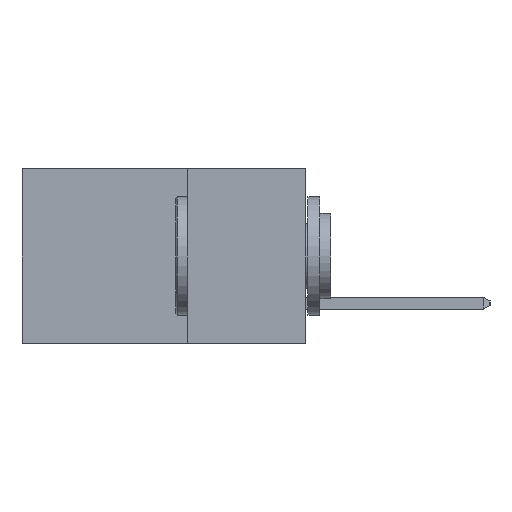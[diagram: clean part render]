
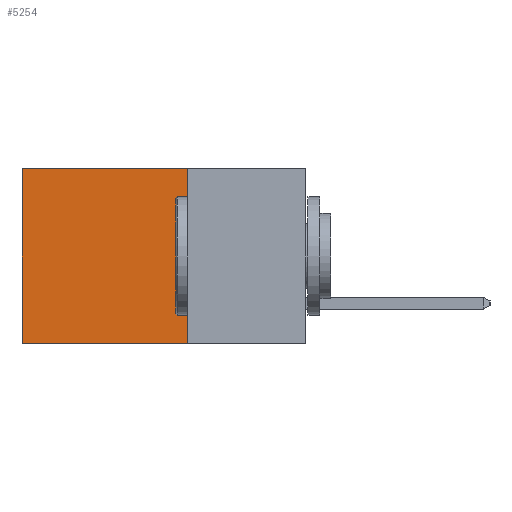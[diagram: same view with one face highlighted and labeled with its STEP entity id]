
A CAD part, left-side view. The second image highlights one B-rep face of the part: STEP entity #5254.
In plain terms, the highlighted planar face has unit normal (-1, 0, 0).
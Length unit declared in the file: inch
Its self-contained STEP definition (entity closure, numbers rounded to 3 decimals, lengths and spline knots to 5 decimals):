
#46 = CARTESIAN_POINT ( 'NONE',  ( 0.2615, 0.6, -0.37 ) ) ;
#59 = CARTESIAN_POINT ( 'NONE',  ( 0.2615, 0.25, 0. ) ) ;
#62 = DIRECTION ( 'NONE',  ( 0., 0., -1. ) ) ;
#90 = LINE ( 'NONE', #10344, #10865 ) ;
#105 = DIRECTION ( 'NONE',  ( 0., 1., 0. ) ) ;
#161 = DIRECTION ( 'NONE',  ( 1., 0., 0. ) ) ;
#405 = EDGE_LOOP ( 'NONE', ( #10939, #8614, #11248, #3374 ) ) ;
#822 = VECTOR ( 'NONE', #105, 39.37008 ) ;
#895 = VECTOR ( 'NONE', #6299, 39.37008 ) ;
#998 = PLANE ( 'NONE',  #1744 ) ;
#1107 = DIRECTION ( 'NONE',  ( 0., 0., -1. ) ) ;
#1227 = CARTESIAN_POINT ( 'NONE',  ( 0.2615, 0.25, -0.37 ) ) ;
#1744 = AXIS2_PLACEMENT_3D ( 'NONE', #1227, #161, #62 ) ;
#3213 = VERTEX_POINT ( 'NONE', #11982 ) ;
#3374 = ORIENTED_EDGE ( 'NONE', *, *, #8757, .T. ) ;
#4241 = CARTESIAN_POINT ( 'NONE',  ( 0.2615, 0.25, -0.37 ) ) ;
#5219 = VERTEX_POINT ( 'NONE', #4241 ) ;
#5245 = CARTESIAN_POINT ( 'NONE',  ( 0.2615, 0.25, -0.37 ) ) ;
#5254 = ADVANCED_FACE ( 'NONE', ( #10800 ), #998, .F. ) ;
#5263 = EDGE_CURVE ( 'NONE', #5577, #6019, #5347, .T. ) ;
#5347 = LINE ( 'NONE', #46, #8139 ) ;
#5577 = VERTEX_POINT ( 'NONE', #11206 ) ;
#6019 = VERTEX_POINT ( 'NONE', #8906 ) ;
#6274 = DIRECTION ( 'NONE',  ( 0., 1., 0. ) ) ;
#6299 = DIRECTION ( 'NONE',  ( 0., 0., -1. ) ) ;
#6428 = LINE ( 'NONE', #59, #822 ) ;
#8139 = VECTOR ( 'NONE', #1107, 39.37008 ) ;
#8614 = ORIENTED_EDGE ( 'NONE', *, *, #9294, .F. ) ;
#8757 = EDGE_CURVE ( 'NONE', #3213, #5577, #6428, .T. ) ;
#8906 = CARTESIAN_POINT ( 'NONE',  ( 0.2615, 0.6, -0.37 ) ) ;
#9258 = LINE ( 'NONE', #5245, #895 ) ;
#9294 = EDGE_CURVE ( 'NONE', #5219, #6019, #90, .T. ) ;
#10344 = CARTESIAN_POINT ( 'NONE',  ( 0.2615, 0.25, -0.37 ) ) ;
#10800 = FACE_OUTER_BOUND ( 'NONE', #405, .T. ) ;
#10865 = VECTOR ( 'NONE', #6274, 39.37008 ) ;
#10939 = ORIENTED_EDGE ( 'NONE', *, *, #5263, .T. ) ;
#11206 = CARTESIAN_POINT ( 'NONE',  ( 0.2615, 0.6, 0. ) ) ;
#11248 = ORIENTED_EDGE ( 'NONE', *, *, #11536, .F. ) ;
#11536 = EDGE_CURVE ( 'NONE', #3213, #5219, #9258, .T. ) ;
#11982 = CARTESIAN_POINT ( 'NONE',  ( 0.2615, 0.25, 0. ) ) ;
